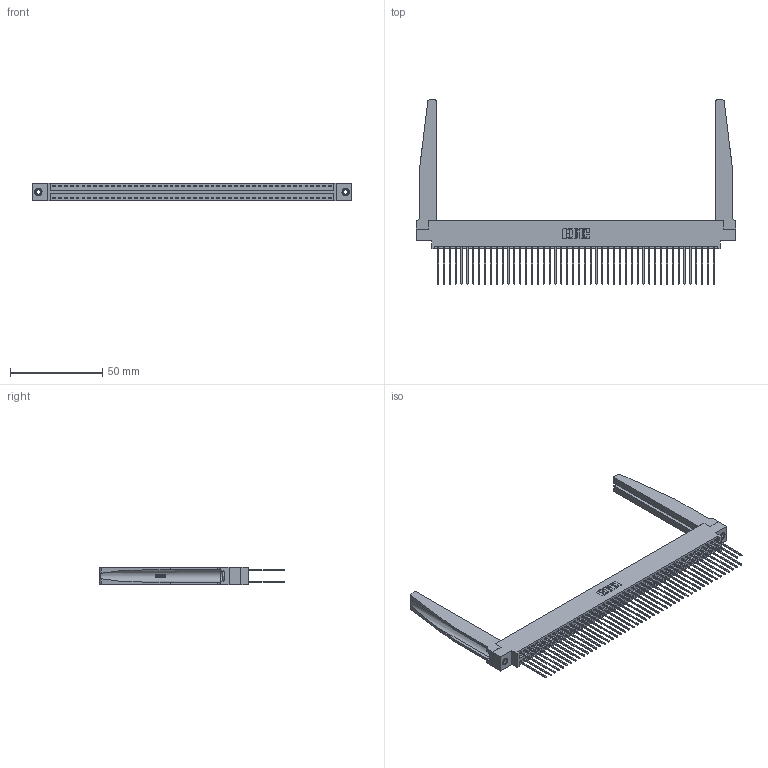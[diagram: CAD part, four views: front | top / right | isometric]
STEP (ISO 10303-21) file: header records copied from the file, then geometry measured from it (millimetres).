
FILE_DESCRIPTION (( 'STEP AP203' ), '1' );
FILE_NAME ('396-096-541-878.STEP', '2019-11-02T16:46:36', ( '' ), ( '' ), 'SwSTEP 2.0', 'SolidWorks 2016', '' );
FILE_SCHEMA (( 'CONFIG_CONTROL_DESIGN' ));
Length unit declared in the file: inch
Products named in the file (5): 346 Part_0.170 Offset - 0.156 Dia-TH; 345-292-001_345-293-141; 346-220-078_345-220-078; 345-250-001_345-250-001-102; 396-096-541-878
Assembly tree (101 placements, depth 2):
  396-096-541-878
    346 Part_0.170 Offset - 0.156 Dia-TH
    345-292-001_345-293-141  x96
    346-220-078_345-220-078  x2
    345-250-001_345-250-001-102  x2
Bounding box: 172.97 x 99.57 x 9.4 mm (x, y, z)
Volume: 24218.7 mm3; surface area: 33246.4 mm2
Topology: 101 solids, 101 shells, 5352 faces, 15829 edges, 10414 vertices
Faces by surface type: plane 3582, cylinder 1718, bspline 36, cone 12, torus 4
Entity records: 35416 total; most frequent: CARTESIAN_POINT 6767, ORIENTED_EDGE 5590, DIRECTION 5001, EDGE_CURVE 2795, VECTOR 2377, LINE 2377, VERTEX_POINT 1856, AXIS2_PLACEMENT_3D 1312
